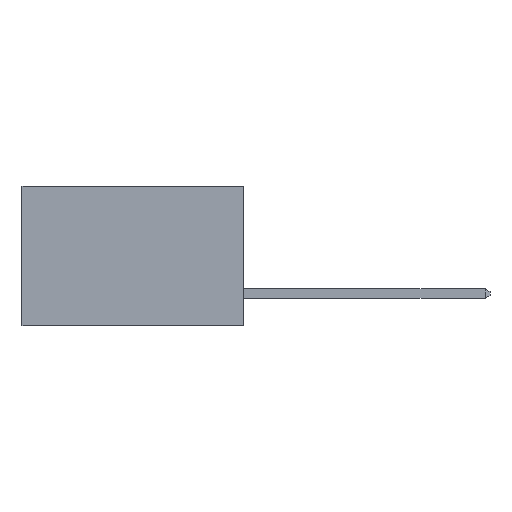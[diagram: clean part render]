
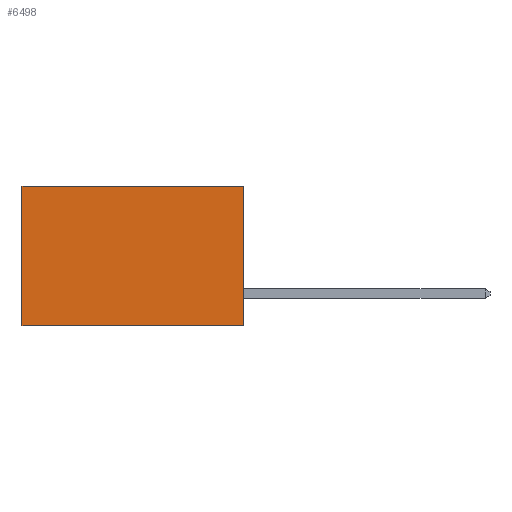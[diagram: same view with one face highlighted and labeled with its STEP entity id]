
A CAD part, left-side view. The second image highlights one B-rep face of the part: STEP entity #6498.
In plain terms, the highlighted planar face has unit normal (-1, 0, 0).
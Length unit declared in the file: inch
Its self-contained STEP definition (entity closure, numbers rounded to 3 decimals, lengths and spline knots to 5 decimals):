
#94 = VECTOR ( 'NONE', #7825, 39.37008 ) ;
#174 = CARTESIAN_POINT ( 'NONE',  ( 0.277, 0.59, 0. ) ) ;
#729 = CARTESIAN_POINT ( 'NONE',  ( 0.277, 0.59, -0.37 ) ) ;
#956 = VERTEX_POINT ( 'NONE', #10792 ) ;
#958 = DIRECTION ( 'NONE',  ( 0., 0., -1. ) ) ;
#978 = AXIS2_PLACEMENT_3D ( 'NONE', #6327, #5867, #5774 ) ;
#1078 = EDGE_CURVE ( 'NONE', #3773, #956, #7182, .T. ) ;
#1143 = EDGE_CURVE ( 'NONE', #3432, #956, #1809, .T. ) ;
#1384 = CARTESIAN_POINT ( 'NONE',  ( 0.277, 0., -0.37 ) ) ;
#1554 = EDGE_CURVE ( 'NONE', #7112, #3773, #2360, .T. ) ;
#1679 = DIRECTION ( 'NONE',  ( 0., 1., 0. ) ) ;
#1809 = LINE ( 'NONE', #729, #6110 ) ;
#2360 = LINE ( 'NONE', #5484, #4054 ) ;
#3432 = VERTEX_POINT ( 'NONE', #174 ) ;
#3773 = VERTEX_POINT ( 'NONE', #1384 ) ;
#4054 = VECTOR ( 'NONE', #4836, 39.37008 ) ;
#4836 = DIRECTION ( 'NONE',  ( 0., 0., -1. ) ) ;
#5484 = CARTESIAN_POINT ( 'NONE',  ( 0.277, 0., -0.37 ) ) ;
#5617 = EDGE_CURVE ( 'NONE', #7112, #3432, #7056, .T. ) ;
#5774 = DIRECTION ( 'NONE',  ( 0., 0., -1. ) ) ;
#5839 = PLANE ( 'NONE',  #978 ) ;
#5867 = DIRECTION ( 'NONE',  ( 1., 0., 0. ) ) ;
#6110 = VECTOR ( 'NONE', #958, 39.37008 ) ;
#6155 = EDGE_LOOP ( 'NONE', ( #6637, #6715, #6842, #6895 ) ) ;
#6327 = CARTESIAN_POINT ( 'NONE',  ( 0.277, 0., -0.37 ) ) ;
#6498 = ADVANCED_FACE ( 'NONE', ( #10127 ), #5839, .F. ) ;
#6637 = ORIENTED_EDGE ( 'NONE', *, *, #1143, .T. ) ;
#6715 = ORIENTED_EDGE ( 'NONE', *, *, #1078, .F. ) ;
#6842 = ORIENTED_EDGE ( 'NONE', *, *, #1554, .F. ) ;
#6895 = ORIENTED_EDGE ( 'NONE', *, *, #5617, .T. ) ;
#7056 = LINE ( 'NONE', #7862, #94 ) ;
#7112 = VERTEX_POINT ( 'NONE', #9877 ) ;
#7182 = LINE ( 'NONE', #7375, #9112 ) ;
#7375 = CARTESIAN_POINT ( 'NONE',  ( 0.277, 0., -0.37 ) ) ;
#7825 = DIRECTION ( 'NONE',  ( 0., 1., 0. ) ) ;
#7862 = CARTESIAN_POINT ( 'NONE',  ( 0.277, 0., 0. ) ) ;
#9112 = VECTOR ( 'NONE', #1679, 39.37008 ) ;
#9877 = CARTESIAN_POINT ( 'NONE',  ( 0.277, 0., 0. ) ) ;
#10127 = FACE_OUTER_BOUND ( 'NONE', #6155, .T. ) ;
#10792 = CARTESIAN_POINT ( 'NONE',  ( 0.277, 0.59, -0.37 ) ) ;
